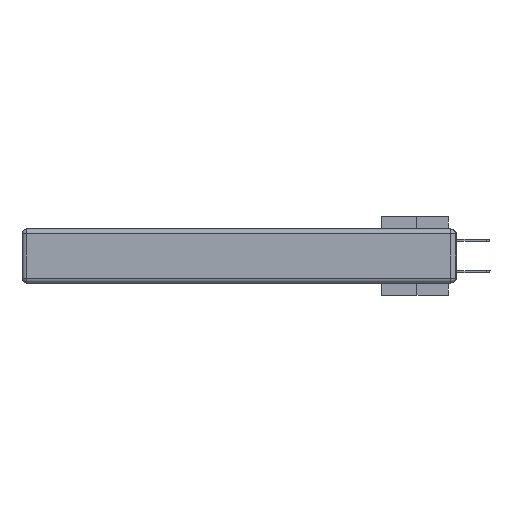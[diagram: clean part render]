
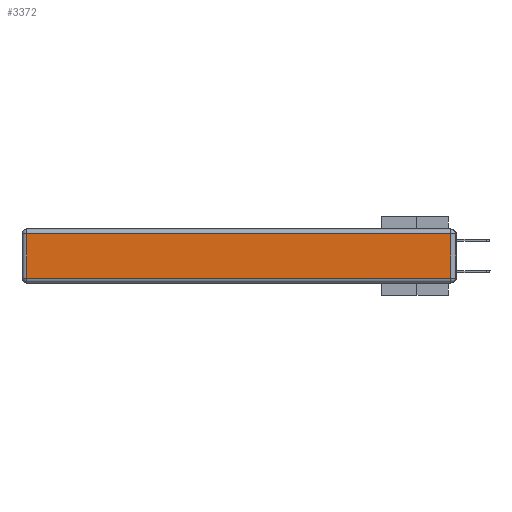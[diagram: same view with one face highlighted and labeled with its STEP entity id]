
A CAD part, left-side view. The second image highlights one B-rep face of the part: STEP entity #3372.
In plain terms, the highlighted planar face has unit normal (-1, 0, 0).
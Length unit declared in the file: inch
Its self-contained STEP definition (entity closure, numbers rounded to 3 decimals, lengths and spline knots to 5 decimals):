
#248 = VECTOR ( 'NONE', #23082, 39.37008 ) ;
#635 = CARTESIAN_POINT ( 'NONE',  ( 0., 0.03, -0.313 ) ) ;
#1492 = FACE_OUTER_BOUND ( 'NONE', #3214, .T. ) ;
#3008 = LINE ( 'NONE', #12512, #3646 ) ;
#3124 = CARTESIAN_POINT ( 'NONE',  ( 0., 2.72, -0.313 ) ) ;
#3214 = EDGE_LOOP ( 'NONE', ( #4384, #24444, #13813, #27935 ) ) ;
#3372 = ADVANCED_FACE ( 'NONE', ( #1492 ), #23258, .T. ) ;
#3646 = VECTOR ( 'NONE', #22109, 39.37008 ) ;
#4309 = DIRECTION ( 'NONE',  ( 0., -1., 0. ) ) ;
#4384 = ORIENTED_EDGE ( 'NONE', *, *, #6519, .T. ) ;
#4406 = LINE ( 'NONE', #30717, #12504 ) ;
#5944 = AXIS2_PLACEMENT_3D ( 'NONE', #8825, #30457, #25580 ) ;
#6519 = EDGE_CURVE ( 'NONE', #7629, #24731, #6954, .T. ) ;
#6954 = LINE ( 'NONE', #28076, #11847 ) ;
#7629 = VERTEX_POINT ( 'NONE', #3124 ) ;
#8825 = CARTESIAN_POINT ( 'NONE',  ( 0., 0., -0.343 ) ) ;
#11623 = CARTESIAN_POINT ( 'NONE',  ( 0., 2.72, -0.03 ) ) ;
#11847 = VECTOR ( 'NONE', #4309, 39.37008 ) ;
#12504 = VECTOR ( 'NONE', #24241, 39.37008 ) ;
#12512 = CARTESIAN_POINT ( 'NONE',  ( 0., 2.72, -0.343 ) ) ;
#13511 = LINE ( 'NONE', #27445, #248 ) ;
#13813 = ORIENTED_EDGE ( 'NONE', *, *, #14241, .T. ) ;
#14241 = EDGE_CURVE ( 'NONE', #30417, #16193, #4406, .T. ) ;
#16193 = VERTEX_POINT ( 'NONE', #11623 ) ;
#16695 = EDGE_CURVE ( 'NONE', #16193, #7629, #3008, .T. ) ;
#22109 = DIRECTION ( 'NONE',  ( 0., 0., -1. ) ) ;
#23082 = DIRECTION ( 'NONE',  ( 0., 0., 1. ) ) ;
#23258 = PLANE ( 'NONE',  #5944 ) ;
#24241 = DIRECTION ( 'NONE',  ( 0., 1., 0. ) ) ;
#24444 = ORIENTED_EDGE ( 'NONE', *, *, #25829, .T. ) ;
#24731 = VERTEX_POINT ( 'NONE', #635 ) ;
#25580 = DIRECTION ( 'NONE',  ( 0., 0., 1. ) ) ;
#25829 = EDGE_CURVE ( 'NONE', #24731, #30417, #13511, .T. ) ;
#26696 = CARTESIAN_POINT ( 'NONE',  ( 0., 0.03, -0.03 ) ) ;
#27445 = CARTESIAN_POINT ( 'NONE',  ( 0., 0.03, -0.343 ) ) ;
#27935 = ORIENTED_EDGE ( 'NONE', *, *, #16695, .T. ) ;
#28076 = CARTESIAN_POINT ( 'NONE',  ( 0., 0., -0.313 ) ) ;
#30417 = VERTEX_POINT ( 'NONE', #26696 ) ;
#30457 = DIRECTION ( 'NONE',  ( -1., 0., 0. ) ) ;
#30717 = CARTESIAN_POINT ( 'NONE',  ( 0., 2.75, -0.03 ) ) ;
